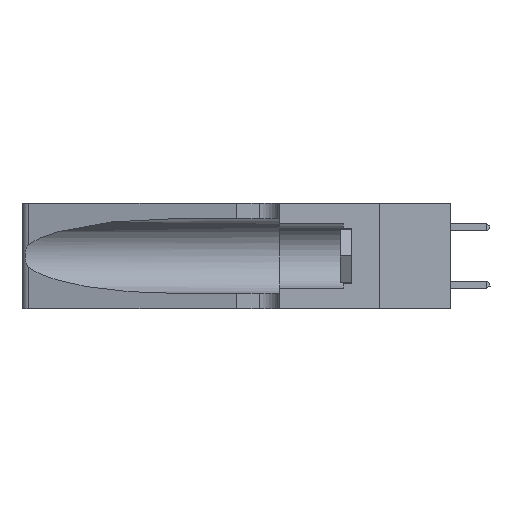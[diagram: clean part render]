
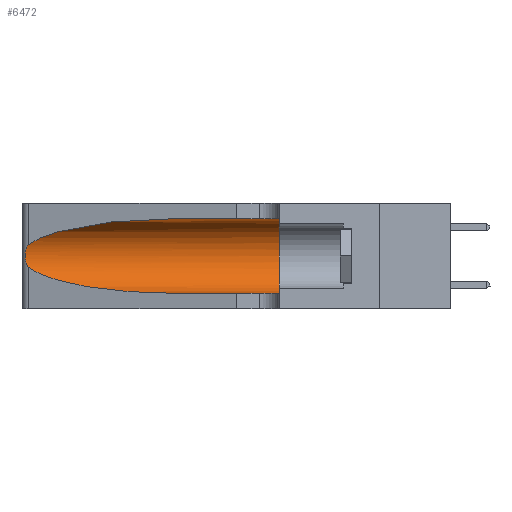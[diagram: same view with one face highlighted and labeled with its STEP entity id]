
A CAD part, left-side view. The second image highlights one B-rep face of the part: STEP entity #6472.
In plain terms, the highlighted cylindrical face has radius 3.308 mm (diameter 6.617 mm), a partial arc.
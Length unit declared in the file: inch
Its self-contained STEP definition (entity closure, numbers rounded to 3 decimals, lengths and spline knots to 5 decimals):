
#221 = EDGE_CURVE ( 'NONE', #16444, #10933, #26509, .T. ) ;
#265 = ORIENTED_EDGE ( 'NONE', *, *, #11401, .F. ) ;
#519 = CARTESIAN_POINT ( 'NONE',  ( 0.1305, 0.35, 0.05475 ) ) ;
#2894 = CARTESIAN_POINT ( 'NONE',  ( 0.25854, 1.2359, 0.20912 ) ) ;
#2937 = CARTESIAN_POINT ( 'NONE',  ( 0.1305, 0.35, 0.185 ) ) ;
#4631 = CARTESIAN_POINT ( 'NONE',  ( 0.18966, 0.96281, 0.31525 ) ) ;
#6329 = CARTESIAN_POINT ( 'NONE',  ( 0.26075, 1.23896, 0.19203 ) ) ;
#6371 = DIRECTION ( 'NONE',  ( 0., 0., 1. ) ) ;
#6472 = ADVANCED_FACE ( 'NONE', ( #43042 ), #33068, .F. ) ;
#7314 = EDGE_CURVE ( 'NONE', #38687, #10933, #20360, .T. ) ;
#7990 = CARTESIAN_POINT ( 'NONE',  ( 0.25487, 1.22718, 0.22369 ) ) ;
#9660 = CARTESIAN_POINT ( 'NONE',  ( 0.26017, 1.23833, 0.17102 ) ) ;
#10206 = CARTESIAN_POINT ( 'NONE',  ( 0.1305, 0.35, 0.31525 ) ) ;
#10419 = CARTESIAN_POINT ( 'NONE',  ( 0.25487, 1.22718, 0.14631 ) ) ;
#10816 = AXIS2_PLACEMENT_3D ( 'NONE', #2937, #26524, #6371 ) ;
#10933 = VERTEX_POINT ( 'NONE', #519 ) ;
#11225 = CARTESIAN_POINT ( 'NONE',  ( 0.1305, 0.72297, 0.31525 ) ) ;
#11401 = EDGE_CURVE ( 'NONE', #40674, #38687, #18494, .T. ) ;
#12108 = ORIENTED_EDGE ( 'NONE', *, *, #7314, .F. ) ;
#13081 = CARTESIAN_POINT ( 'NONE',  ( 0.25789, 1.23486, 0.15765 ) ) ;
#13102 = CARTESIAN_POINT ( 'NONE',  ( 0.1305, 1.61858, 0.31525 ) ) ;
#13981 = CARTESIAN_POINT ( 'NONE',  ( 0.1305, 0.72297, 0.05475 ) ) ;
#15658 = ORIENTED_EDGE ( 'NONE', *, *, #25635, .T. ) ;
#16352 = CARTESIAN_POINT ( 'NONE',  ( 0.25487, 1.22718, 0.22369 ) ) ;
#16375 =( BOUNDED_CURVE ( )  B_SPLINE_CURVE ( 3, ( #11225, #4631, #28152, #7990 ),
 .UNSPECIFIED., .F., .F. ) 
 B_SPLINE_CURVE_WITH_KNOTS ( ( 4, 4 ),
 ( 1.5708, 2.84003 ),
 .UNSPECIFIED. ) 
 CURVE ( )  GEOMETRIC_REPRESENTATION_ITEM ( )  RATIONAL_B_SPLINE_CURVE ( ( 1., 0.87, 0.87, 1. ) ) 
 REPRESENTATION_ITEM ( '' )  );
#16444 = VERTEX_POINT ( 'NONE', #17047 ) ;
#16493 = CARTESIAN_POINT ( 'NONE',  ( 0.25555, 1.22993, 0.14849 ) ) ;
#16508 = DIRECTION ( 'NONE',  ( 0., -1., 0. ) ) ;
#17047 = CARTESIAN_POINT ( 'NONE',  ( 0.1305, 0.72297, 0.05475 ) ) ;
#17536 = EDGE_LOOP ( 'NONE', ( #15658, #25547, #40028, #30689, #12108, #265 ) ) ;
#17573 = VECTOR ( 'NONE', #28910, 39.37008 ) ;
#18494 = LINE ( 'NONE', #13102, #35229 ) ;
#18981 = DIRECTION ( 'NONE',  ( 0., -1., 0. ) ) ;
#20360 = CIRCLE ( 'NONE', #10816, 0.13025 ) ;
#20500 = VERTEX_POINT ( 'NONE', #38957 ) ;
#20935 =( BOUNDED_CURVE ( )  B_SPLINE_CURVE ( 3, ( #10419, #40645, #34062, #13981 ),
 .UNSPECIFIED., .F., .F. ) 
 B_SPLINE_CURVE_WITH_KNOTS ( ( 4, 4 ),
 ( 3.44316, 4.71239 ),
 .UNSPECIFIED. ) 
 CURVE ( )  GEOMETRIC_REPRESENTATION_ITEM ( )  RATIONAL_B_SPLINE_CURVE ( ( 1., 0.87, 0.87, 1. ) ) 
 REPRESENTATION_ITEM ( '' )  );
#22249 = EDGE_CURVE ( 'NONE', #20500, #32224, #31950, .T. ) ;
#23078 = CARTESIAN_POINT ( 'NONE',  ( 0.25787, 1.23484, 0.2124 ) ) ;
#24754 = CARTESIAN_POINT ( 'NONE',  ( 0.1305, 0.72297, 0.31525 ) ) ;
#25547 = ORIENTED_EDGE ( 'NONE', *, *, #22249, .T. ) ;
#25562 = CARTESIAN_POINT ( 'NONE',  ( 0.1305, 1.61858, 0.05475 ) ) ;
#25635 = EDGE_CURVE ( 'NONE', #40674, #20500, #16375, .T. ) ;
#26478 = CARTESIAN_POINT ( 'NONE',  ( 0.26018, 1.23835, 0.19895 ) ) ;
#26509 = LINE ( 'NONE', #25562, #17573 ) ;
#26524 = DIRECTION ( 'NONE',  ( 0., 1., 0. ) ) ;
#28152 = CARTESIAN_POINT ( 'NONE',  ( 0.2373, 1.15595, 0.28018 ) ) ;
#28910 = DIRECTION ( 'NONE',  ( 0., -1., 0. ) ) ;
#28920 = CARTESIAN_POINT ( 'NONE',  ( 0.1305, 1.61858, 0.185 ) ) ;
#29815 = CARTESIAN_POINT ( 'NONE',  ( 0.26075, 1.23896, 0.178 ) ) ;
#30689 = ORIENTED_EDGE ( 'NONE', *, *, #221, .T. ) ;
#31950 = B_SPLINE_CURVE_WITH_KNOTS ( 'NONE', 3,
 ( #16352, #39757, #43159, #23078, #2894, #26478, #6329, #29815, #9660, #33183, #13081, #36536, #16493, #39908 ),
 .UNSPECIFIED., .F., .F.,
 ( 4, 2, 2, 2, 2, 2, 4 ),
 ( 0., 0.00027, 0.00053, 0.00107, 0.0016, 0.00187, 0.00214 ),
 .UNSPECIFIED. ) ;
#32224 = VERTEX_POINT ( 'NONE', #39848 ) ;
#33068 = CYLINDRICAL_SURFACE ( 'NONE', #42613, 0.13025 ) ;
#33183 = CARTESIAN_POINT ( 'NONE',  ( 0.25856, 1.23593, 0.16098 ) ) ;
#34062 = CARTESIAN_POINT ( 'NONE',  ( 0.18966, 0.96281, 0.05475 ) ) ;
#35229 = VECTOR ( 'NONE', #16508, 39.37008 ) ;
#36536 = CARTESIAN_POINT ( 'NONE',  ( 0.25639, 1.23186, 0.15144 ) ) ;
#38687 = VERTEX_POINT ( 'NONE', #10206 ) ;
#38957 = CARTESIAN_POINT ( 'NONE',  ( 0.25487, 1.22718, 0.22369 ) ) ;
#39757 = CARTESIAN_POINT ( 'NONE',  ( 0.25555, 1.22994, 0.2215 ) ) ;
#39848 = CARTESIAN_POINT ( 'NONE',  ( 0.25487, 1.22718, 0.14631 ) ) ;
#39908 = CARTESIAN_POINT ( 'NONE',  ( 0.25487, 1.22718, 0.14631 ) ) ;
#40028 = ORIENTED_EDGE ( 'NONE', *, *, #41166, .T. ) ;
#40645 = CARTESIAN_POINT ( 'NONE',  ( 0.2373, 1.15595, 0.08982 ) ) ;
#40674 = VERTEX_POINT ( 'NONE', #24754 ) ;
#41166 = EDGE_CURVE ( 'NONE', #32224, #16444, #20935, .T. ) ;
#42399 = DIRECTION ( 'NONE',  ( 0., 0., -1. ) ) ;
#42613 = AXIS2_PLACEMENT_3D ( 'NONE', #28920, #18981, #42399 ) ;
#43042 = FACE_OUTER_BOUND ( 'NONE', #17536, .T. ) ;
#43159 = CARTESIAN_POINT ( 'NONE',  ( 0.25639, 1.23184, 0.21858 ) ) ;
